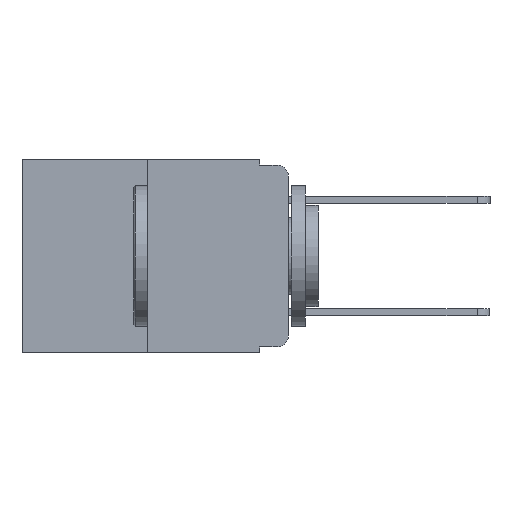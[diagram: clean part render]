
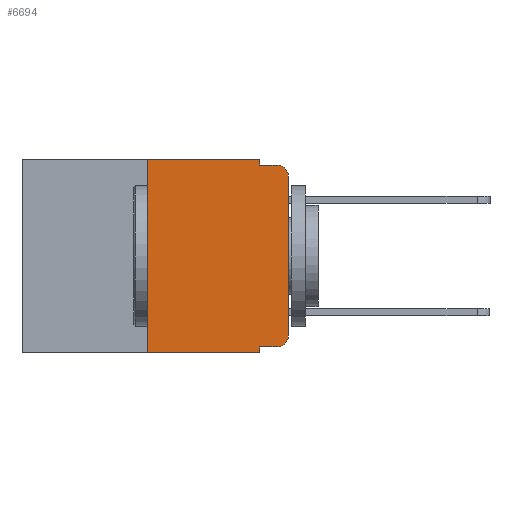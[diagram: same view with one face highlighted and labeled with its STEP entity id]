
A CAD part, left-side view. The second image highlights one B-rep face of the part: STEP entity #6694.
In plain terms, the highlighted planar face has unit normal (-1, 0, 0).
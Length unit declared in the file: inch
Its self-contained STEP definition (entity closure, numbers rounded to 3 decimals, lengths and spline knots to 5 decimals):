
#370 = CARTESIAN_POINT ( 'NONE',  ( 0., 0.051, -0.333 ) ) ;
#513 = VECTOR ( 'NONE', #11914, 39.37008 ) ;
#611 = VERTEX_POINT ( 'NONE', #1114 ) ;
#634 = VERTEX_POINT ( 'NONE', #3020 ) ;
#877 = CIRCLE ( 'NONE', #3715, 0.02 ) ;
#1114 = CARTESIAN_POINT ( 'NONE',  ( 0., 0.051, -0.343 ) ) ;
#1485 = DIRECTION ( 'NONE',  ( 0., 0., -1. ) ) ;
#1501 = ORIENTED_EDGE ( 'NONE', *, *, #8215, .F. ) ;
#1953 = DIRECTION ( 'NONE',  ( 0., -1., 0. ) ) ;
#1990 = PLANE ( 'NONE',  #8938 ) ;
#2282 = CARTESIAN_POINT ( 'NONE',  ( 0., 0., -0.313 ) ) ;
#2369 = DIRECTION ( 'NONE',  ( -1., 0., 0. ) ) ;
#2381 = VERTEX_POINT ( 'NONE', #6010 ) ;
#2443 = EDGE_CURVE ( 'NONE', #6619, #611, #11531, .T. ) ;
#2741 = EDGE_CURVE ( 'NONE', #6721, #2381, #11110, .T. ) ;
#2743 = ORIENTED_EDGE ( 'NONE', *, *, #9888, .F. ) ;
#2949 = VECTOR ( 'NONE', #1485, 39.37008 ) ;
#3020 = CARTESIAN_POINT ( 'NONE',  ( 0., 0.051, 0. ) ) ;
#3486 = CARTESIAN_POINT ( 'NONE',  ( 0., 0., -0.03 ) ) ;
#3538 = DIRECTION ( 'NONE',  ( 0., -1., 0. ) ) ;
#3545 = VECTOR ( 'NONE', #3538, 39.37008 ) ;
#3715 = AXIS2_PLACEMENT_3D ( 'NONE', #9129, #2369, #5090 ) ;
#3814 = ORIENTED_EDGE ( 'NONE', *, *, #4745, .T. ) ;
#3960 = VECTOR ( 'NONE', #6795, 39.37008 ) ;
#3977 = CARTESIAN_POINT ( 'NONE',  ( 0., 0.473, 0. ) ) ;
#3992 = ORIENTED_EDGE ( 'NONE', *, *, #8926, .T. ) ;
#4082 = EDGE_CURVE ( 'NONE', #5098, #2381, #877, .T. ) ;
#4091 = VECTOR ( 'NONE', #1953, 39.37008 ) ;
#4274 = LINE ( 'NONE', #7723, #3960 ) ;
#4378 = FACE_OUTER_BOUND ( 'NONE', #11205, .T. ) ;
#4702 = DIRECTION ( 'NONE',  ( -1., 0., 0. ) ) ;
#4722 = VECTOR ( 'NONE', #6060, 39.37008 ) ;
#4745 = EDGE_CURVE ( 'NONE', #8665, #5098, #4274, .T. ) ;
#4896 = CARTESIAN_POINT ( 'NONE',  ( 0., 0.051, -0.01 ) ) ;
#4973 = DIRECTION ( 'NONE',  ( 0., 0., -1. ) ) ;
#5090 = DIRECTION ( 'NONE',  ( 0., 0., -1. ) ) ;
#5098 = VERTEX_POINT ( 'NONE', #3486 ) ;
#5377 = CARTESIAN_POINT ( 'NONE',  ( 0., 0.051, 0. ) ) ;
#5690 = LINE ( 'NONE', #370, #10502 ) ;
#6010 = CARTESIAN_POINT ( 'NONE',  ( 0., 0.02, -0.01 ) ) ;
#6060 = DIRECTION ( 'NONE',  ( 0., 0., -1. ) ) ;
#6168 = LINE ( 'NONE', #5377, #2949 ) ;
#6243 = DIRECTION ( 'NONE',  ( 0., -1., 0. ) ) ;
#6351 = CARTESIAN_POINT ( 'NONE',  ( 0., 0.473, -0.343 ) ) ;
#6619 = VERTEX_POINT ( 'NONE', #11196 ) ;
#6694 = ADVANCED_FACE ( 'NONE', ( #4378 ), #1990, .F. ) ;
#6721 = VERTEX_POINT ( 'NONE', #11349 ) ;
#6795 = DIRECTION ( 'NONE',  ( 0., 0., 1. ) ) ;
#7280 = DIRECTION ( 'NONE',  ( 0., -1., 0. ) ) ;
#7528 = LINE ( 'NONE', #11431, #4722 ) ;
#7534 = CARTESIAN_POINT ( 'NONE',  ( 0., 0.25, 0. ) ) ;
#7571 = ORIENTED_EDGE ( 'NONE', *, *, #2443, .T. ) ;
#7665 = VERTEX_POINT ( 'NONE', #9242 ) ;
#7676 = CARTESIAN_POINT ( 'NONE',  ( 0., 0.25, 0. ) ) ;
#7723 = CARTESIAN_POINT ( 'NONE',  ( 0., 0., 0. ) ) ;
#7743 = AXIS2_PLACEMENT_3D ( 'NONE', #10176, #4702, #11059 ) ;
#8215 = EDGE_CURVE ( 'NONE', #8432, #634, #8559, .T. ) ;
#8295 = CIRCLE ( 'NONE', #7743, 0.02 ) ;
#8432 = VERTEX_POINT ( 'NONE', #7676 ) ;
#8559 = LINE ( 'NONE', #10913, #3545 ) ;
#8665 = VERTEX_POINT ( 'NONE', #2282 ) ;
#8705 = EDGE_CURVE ( 'NONE', #7665, #9008, #5690, .T. ) ;
#8926 = EDGE_CURVE ( 'NONE', #9008, #8665, #8295, .T. ) ;
#8938 = AXIS2_PLACEMENT_3D ( 'NONE', #3977, #10430, #4973 ) ;
#9008 = VERTEX_POINT ( 'NONE', #11137 ) ;
#9129 = CARTESIAN_POINT ( 'NONE',  ( 0., 0.02, -0.03 ) ) ;
#9186 = VECTOR ( 'NONE', #7280, 39.37008 ) ;
#9242 = CARTESIAN_POINT ( 'NONE',  ( 0., 0.051, -0.333 ) ) ;
#9786 = ORIENTED_EDGE ( 'NONE', *, *, #11650, .F. ) ;
#9888 = EDGE_CURVE ( 'NONE', #7665, #611, #7528, .T. ) ;
#10176 = CARTESIAN_POINT ( 'NONE',  ( 0., 0.02, -0.313 ) ) ;
#10430 = DIRECTION ( 'NONE',  ( 1., 0., 0. ) ) ;
#10473 = EDGE_CURVE ( 'NONE', #6619, #8432, #10555, .T. ) ;
#10502 = VECTOR ( 'NONE', #6243, 39.37008 ) ;
#10555 = LINE ( 'NONE', #7534, #513 ) ;
#10741 = ORIENTED_EDGE ( 'NONE', *, *, #8705, .T. ) ;
#10913 = CARTESIAN_POINT ( 'NONE',  ( 0., 0.473, 0. ) ) ;
#11012 = ORIENTED_EDGE ( 'NONE', *, *, #2741, .F. ) ;
#11059 = DIRECTION ( 'NONE',  ( 0., 0., -1. ) ) ;
#11110 = LINE ( 'NONE', #4896, #4091 ) ;
#11137 = CARTESIAN_POINT ( 'NONE',  ( 0., 0.02, -0.333 ) ) ;
#11196 = CARTESIAN_POINT ( 'NONE',  ( 0., 0.25, -0.343 ) ) ;
#11205 = EDGE_LOOP ( 'NONE', ( #3814, #11428, #11012, #9786, #1501, #11441, #7571, #2743, #10741, #3992 ) ) ;
#11349 = CARTESIAN_POINT ( 'NONE',  ( 0., 0.051, -0.01 ) ) ;
#11428 = ORIENTED_EDGE ( 'NONE', *, *, #4082, .T. ) ;
#11431 = CARTESIAN_POINT ( 'NONE',  ( 0., 0.051, 0. ) ) ;
#11441 = ORIENTED_EDGE ( 'NONE', *, *, #10473, .F. ) ;
#11531 = LINE ( 'NONE', #6351, #9186 ) ;
#11650 = EDGE_CURVE ( 'NONE', #634, #6721, #6168, .T. ) ;
#11914 = DIRECTION ( 'NONE',  ( 0., 0., 1. ) ) ;
